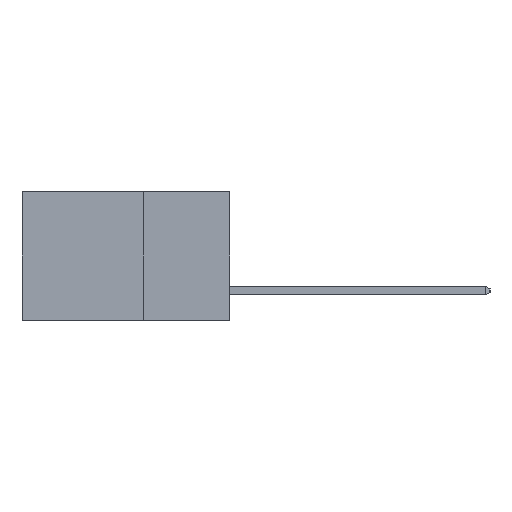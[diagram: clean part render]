
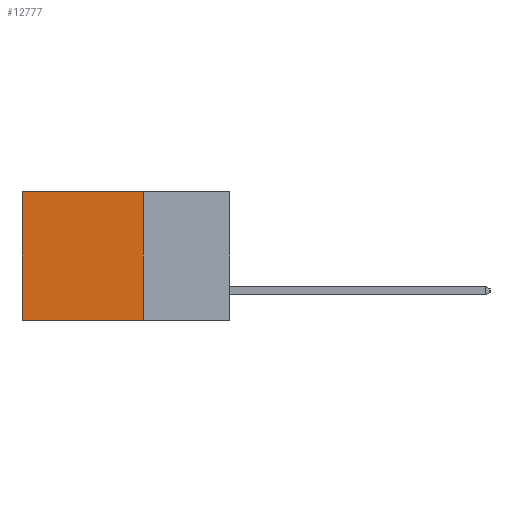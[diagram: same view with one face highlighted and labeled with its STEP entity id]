
A CAD part, left-side view. The second image highlights one B-rep face of the part: STEP entity #12777.
In plain terms, the highlighted planar face has unit normal (-1, 0, 0).
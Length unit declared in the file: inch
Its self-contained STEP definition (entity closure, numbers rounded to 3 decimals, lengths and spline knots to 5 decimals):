
#429 = LINE ( 'NONE', #11329, #10478 ) ;
#813 = DIRECTION ( 'NONE',  ( 0., 1., 0. ) ) ;
#955 = DIRECTION ( 'NONE',  ( 1., 0., 0. ) ) ;
#2095 = VERTEX_POINT ( 'NONE', #13957 ) ;
#6026 = CARTESIAN_POINT ( 'NONE',  ( 0.298, 0.25, 0. ) ) ;
#6226 = VECTOR ( 'NONE', #23828, 39.37008 ) ;
#6337 = ORIENTED_EDGE ( 'NONE', *, *, #22222, .T. ) ;
#6675 = VERTEX_POINT ( 'NONE', #12319 ) ;
#6720 = ORIENTED_EDGE ( 'NONE', *, *, #10401, .F. ) ;
#6868 = LINE ( 'NONE', #6026, #6226 ) ;
#7103 = VERTEX_POINT ( 'NONE', #7585 ) ;
#7585 = CARTESIAN_POINT ( 'NONE',  ( 0.298, 0.6, -0.37 ) ) ;
#8039 = EDGE_CURVE ( 'NONE', #2095, #18926, #6868, .T. ) ;
#8451 = ORIENTED_EDGE ( 'NONE', *, *, #8039, .F. ) ;
#9216 = LINE ( 'NONE', #10875, #15013 ) ;
#10290 = EDGE_CURVE ( 'NONE', #2095, #6675, #18240, .T. ) ;
#10401 = EDGE_CURVE ( 'NONE', #18926, #7103, #429, .T. ) ;
#10478 = VECTOR ( 'NONE', #21215, 39.37008 ) ;
#10875 = CARTESIAN_POINT ( 'NONE',  ( 0.298, 0.6, 0. ) ) ;
#11329 = CARTESIAN_POINT ( 'NONE',  ( 0.298, 0.25, -0.37 ) ) ;
#12319 = CARTESIAN_POINT ( 'NONE',  ( 0.298, 0.6, 0. ) ) ;
#12777 = ADVANCED_FACE ( 'NONE', ( #15038 ), #18836, .F. ) ;
#12986 = CARTESIAN_POINT ( 'NONE',  ( 0.298, 0.25, 0. ) ) ;
#12996 = VECTOR ( 'NONE', #813, 39.37008 ) ;
#13332 = EDGE_LOOP ( 'NONE', ( #6337, #6720, #8451, #16747 ) ) ;
#13957 = CARTESIAN_POINT ( 'NONE',  ( 0.298, 0.25, 0. ) ) ;
#14966 = DIRECTION ( 'NONE',  ( 0., 0., -1. ) ) ;
#15013 = VECTOR ( 'NONE', #20699, 39.37008 ) ;
#15038 = FACE_OUTER_BOUND ( 'NONE', #13332, .T. ) ;
#16563 = AXIS2_PLACEMENT_3D ( 'NONE', #12986, #955, #14966 ) ;
#16747 = ORIENTED_EDGE ( 'NONE', *, *, #10290, .T. ) ;
#18240 = LINE ( 'NONE', #22510, #12996 ) ;
#18836 = PLANE ( 'NONE',  #16563 ) ;
#18926 = VERTEX_POINT ( 'NONE', #22669 ) ;
#20699 = DIRECTION ( 'NONE',  ( 0., 0., -1. ) ) ;
#21215 = DIRECTION ( 'NONE',  ( 0., 1., 0. ) ) ;
#22222 = EDGE_CURVE ( 'NONE', #6675, #7103, #9216, .T. ) ;
#22510 = CARTESIAN_POINT ( 'NONE',  ( 0.298, 0.25, 0. ) ) ;
#22669 = CARTESIAN_POINT ( 'NONE',  ( 0.298, 0.25, -0.37 ) ) ;
#23828 = DIRECTION ( 'NONE',  ( 0., 0., -1. ) ) ;
